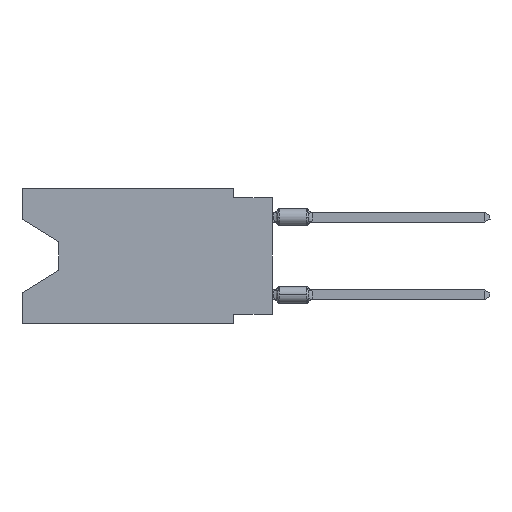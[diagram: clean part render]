
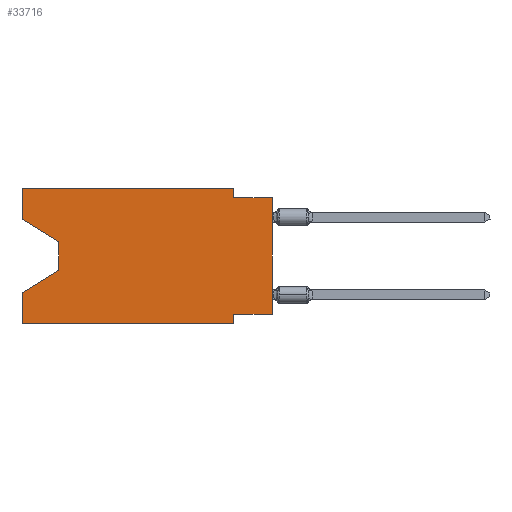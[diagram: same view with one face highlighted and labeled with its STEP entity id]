
A CAD part, left-side view. The second image highlights one B-rep face of the part: STEP entity #33716.
In plain terms, the highlighted planar face has unit normal (-1, 0, 0).
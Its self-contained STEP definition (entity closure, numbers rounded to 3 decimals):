
#106 = CARTESIAN_POINT ( 'NONE',  ( 0., 0., -8.255 ) ) ;
#453 = VECTOR ( 'NONE', #25975, 1000. ) ;
#870 = LINE ( 'NONE', #9242, #20045 ) ;
#1056 = ORIENTED_EDGE ( 'NONE', *, *, #33624, .F. ) ;
#1107 = DIRECTION ( 'NONE',  ( 0., 0.855, -0.519 ) ) ;
#1128 = CARTESIAN_POINT ( 'NONE',  ( 0., 0., -0.635 ) ) ;
#1375 = VERTEX_POINT ( 'NONE', #36576 ) ;
#2446 = VECTOR ( 'NONE', #53870, 1000. ) ;
#2481 = CARTESIAN_POINT ( 'NONE',  ( 0., 16.383, 0. ) ) ;
#4849 = ORIENTED_EDGE ( 'NONE', *, *, #15157, .F. ) ;
#4896 = CARTESIAN_POINT ( 'NONE',  ( 0., 16.383, 0. ) ) ;
#5039 = EDGE_CURVE ( 'NONE', #33933, #32939, #38800, .T. ) ;
#5180 = FACE_OUTER_BOUND ( 'NONE', #18265, .T. ) ;
#5343 = VERTEX_POINT ( 'NONE', #54723 ) ;
#5551 = CARTESIAN_POINT ( 'NONE',  ( 0., 0., -0.635 ) ) ;
#5605 = EDGE_CURVE ( 'NONE', #8811, #1375, #36705, .T. ) ;
#5911 = ORIENTED_EDGE ( 'NONE', *, *, #5605, .T. ) ;
#6388 = EDGE_CURVE ( 'NONE', #50952, #47474, #15059, .T. ) ;
#7209 = CARTESIAN_POINT ( 'NONE',  ( 0., 13.97, -3.505 ) ) ;
#7977 = CARTESIAN_POINT ( 'NONE',  ( 0., 16.383, -8.89 ) ) ;
#8169 = VERTEX_POINT ( 'NONE', #47263 ) ;
#8811 = VERTEX_POINT ( 'NONE', #7209 ) ;
#9111 = DIRECTION ( 'NONE',  ( 0., 0., -1. ) ) ;
#9242 = CARTESIAN_POINT ( 'NONE',  ( 0., 16.383, 0. ) ) ;
#9373 = PLANE ( 'NONE',  #44639 ) ;
#9506 = CARTESIAN_POINT ( 'NONE',  ( 0., 16.383, 0. ) ) ;
#9743 = VECTOR ( 'NONE', #24310, 1000. ) ;
#9767 = CARTESIAN_POINT ( 'NONE',  ( 0., 2.54, -8.89 ) ) ;
#12442 = ORIENTED_EDGE ( 'NONE', *, *, #43058, .T. ) ;
#13051 = ORIENTED_EDGE ( 'NONE', *, *, #5039, .F. ) ;
#14155 = ORIENTED_EDGE ( 'NONE', *, *, #15861, .F. ) ;
#14644 = VECTOR ( 'NONE', #15195, 1000. ) ;
#15059 = LINE ( 'NONE', #2481, #52630 ) ;
#15157 = EDGE_CURVE ( 'NONE', #46656, #37839, #54773, .T. ) ;
#15195 = DIRECTION ( 'NONE',  ( 0., 0., -1. ) ) ;
#15490 = VECTOR ( 'NONE', #44084, 1000. ) ;
#15861 = EDGE_CURVE ( 'NONE', #24876, #39146, #870, .T. ) ;
#16653 = CARTESIAN_POINT ( 'NONE',  ( 0., 16.383, 0. ) ) ;
#18265 = EDGE_LOOP ( 'NONE', ( #39855, #5911, #40390, #38144, #49640, #43016, #4849, #12442, #13051, #49919, #14155, #1056 ) ) ;
#20045 = VECTOR ( 'NONE', #44131, 1000. ) ;
#20633 = LINE ( 'NONE', #30106, #51047 ) ;
#21219 = LINE ( 'NONE', #46653, #453 ) ;
#21381 = VECTOR ( 'NONE', #28369, 1000. ) ;
#22279 = VECTOR ( 'NONE', #37881, 1000. ) ;
#22725 = CARTESIAN_POINT ( 'NONE',  ( 0., 16.383, -8.89 ) ) ;
#23177 = LINE ( 'NONE', #9767, #36675 ) ;
#23667 = CARTESIAN_POINT ( 'NONE',  ( 0., 2.54, 0. ) ) ;
#24190 = LINE ( 'NONE', #7977, #21381 ) ;
#24242 = EDGE_CURVE ( 'NONE', #39146, #33933, #44885, .T. ) ;
#24310 = DIRECTION ( 'NONE',  ( 0., 1., 0. ) ) ;
#24854 = CARTESIAN_POINT ( 'NONE',  ( 0., 0., -8.255 ) ) ;
#24876 = VERTEX_POINT ( 'NONE', #9506 ) ;
#25975 = DIRECTION ( 'NONE',  ( 0., 0., 1. ) ) ;
#27290 = CARTESIAN_POINT ( 'NONE',  ( 0., 2.54, -8.255 ) ) ;
#28369 = DIRECTION ( 'NONE',  ( 0., -1., 0. ) ) ;
#28692 = CARTESIAN_POINT ( 'NONE',  ( 0., 2.54, 0. ) ) ;
#30106 = CARTESIAN_POINT ( 'NONE',  ( 0., 16.383, -2.038 ) ) ;
#30987 = DIRECTION ( 'NONE',  ( 0., 0., -1. ) ) ;
#31764 = VECTOR ( 'NONE', #1107, 1000. ) ;
#32639 = DIRECTION ( 'NONE',  ( 0., 0., 1. ) ) ;
#32939 = VERTEX_POINT ( 'NONE', #1128 ) ;
#32950 = CARTESIAN_POINT ( 'NONE',  ( 0., 16.383, -6.852 ) ) ;
#33624 = EDGE_CURVE ( 'NONE', #5343, #24876, #54692, .T. ) ;
#33716 = ADVANCED_FACE ( 'NONE', ( #5180 ), #9373, .F. ) ;
#33933 = VERTEX_POINT ( 'NONE', #36168 ) ;
#36168 = CARTESIAN_POINT ( 'NONE',  ( 0., 2.54, -0.635 ) ) ;
#36576 = CARTESIAN_POINT ( 'NONE',  ( 0., 13.97, -5.385 ) ) ;
#36675 = VECTOR ( 'NONE', #30987, 1000. ) ;
#36705 = LINE ( 'NONE', #53513, #14644 ) ;
#37601 = EDGE_CURVE ( 'NONE', #5343, #8811, #20633, .T. ) ;
#37839 = VERTEX_POINT ( 'NONE', #27290 ) ;
#37881 = DIRECTION ( 'NONE',  ( 0., 0., 1. ) ) ;
#38144 = ORIENTED_EDGE ( 'NONE', *, *, #6388, .F. ) ;
#38510 = DIRECTION ( 'NONE',  ( 0., -0.855, -0.519 ) ) ;
#38800 = LINE ( 'NONE', #5551, #15490 ) ;
#39146 = VERTEX_POINT ( 'NONE', #28692 ) ;
#39855 = ORIENTED_EDGE ( 'NONE', *, *, #37601, .T. ) ;
#40390 = ORIENTED_EDGE ( 'NONE', *, *, #44412, .T. ) ;
#42070 = EDGE_CURVE ( 'NONE', #50952, #8169, #24190, .T. ) ;
#43016 = ORIENTED_EDGE ( 'NONE', *, *, #52869, .F. ) ;
#43058 = EDGE_CURVE ( 'NONE', #46656, #32939, #21219, .T. ) ;
#44084 = DIRECTION ( 'NONE',  ( 0., -1., 0. ) ) ;
#44131 = DIRECTION ( 'NONE',  ( 0., -1., 0. ) ) ;
#44412 = EDGE_CURVE ( 'NONE', #1375, #47474, #47763, .T. ) ;
#44639 = AXIS2_PLACEMENT_3D ( 'NONE', #4896, #51600, #9111 ) ;
#44669 = CARTESIAN_POINT ( 'NONE',  ( 0., 13.97, -5.385 ) ) ;
#44885 = LINE ( 'NONE', #23667, #2446 ) ;
#46653 = CARTESIAN_POINT ( 'NONE',  ( 0., 0., 0. ) ) ;
#46656 = VERTEX_POINT ( 'NONE', #106 ) ;
#47263 = CARTESIAN_POINT ( 'NONE',  ( 0., 2.54, -8.89 ) ) ;
#47474 = VERTEX_POINT ( 'NONE', #32950 ) ;
#47763 = LINE ( 'NONE', #44669, #31764 ) ;
#49640 = ORIENTED_EDGE ( 'NONE', *, *, #42070, .T. ) ;
#49919 = ORIENTED_EDGE ( 'NONE', *, *, #24242, .F. ) ;
#50952 = VERTEX_POINT ( 'NONE', #22725 ) ;
#51047 = VECTOR ( 'NONE', #38510, 1000. ) ;
#51600 = DIRECTION ( 'NONE',  ( 1., 0., 0. ) ) ;
#52630 = VECTOR ( 'NONE', #32639, 1000. ) ;
#52869 = EDGE_CURVE ( 'NONE', #37839, #8169, #23177, .T. ) ;
#53513 = CARTESIAN_POINT ( 'NONE',  ( 0., 13.97, -3.505 ) ) ;
#53870 = DIRECTION ( 'NONE',  ( 0., 0., -1. ) ) ;
#54692 = LINE ( 'NONE', #16653, #22279 ) ;
#54723 = CARTESIAN_POINT ( 'NONE',  ( 0., 16.383, -2.038 ) ) ;
#54773 = LINE ( 'NONE', #24854, #9743 ) ;
